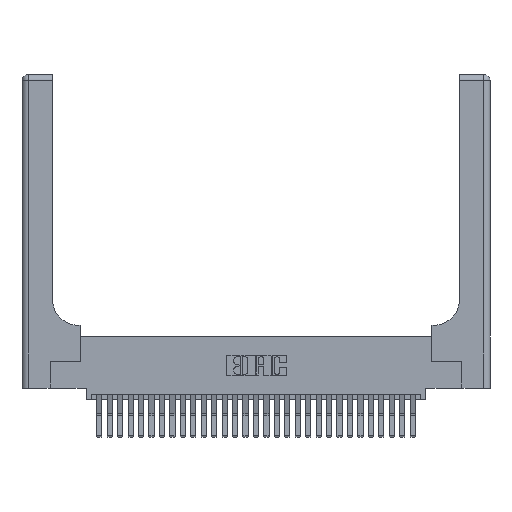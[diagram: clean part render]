
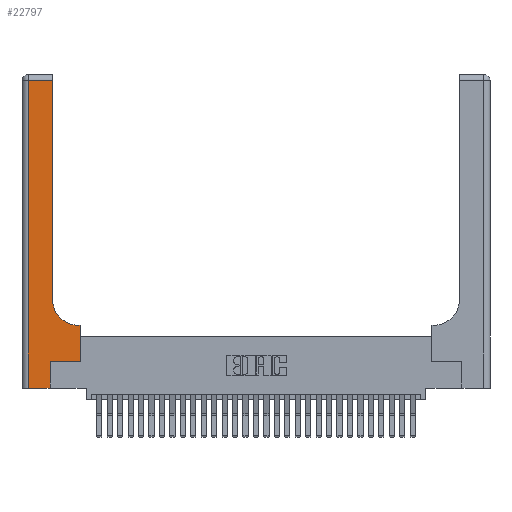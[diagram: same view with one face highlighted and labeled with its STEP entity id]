
A CAD part, top view. The second image highlights one B-rep face of the part: STEP entity #22797.
In plain terms, the highlighted planar face has unit normal (0, 0, 1).
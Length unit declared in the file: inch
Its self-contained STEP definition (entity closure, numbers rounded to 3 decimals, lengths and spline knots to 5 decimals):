
#344 = CARTESIAN_POINT ( 'NONE',  ( 0., 0., 0.37 ) ) ;
#548 = ORIENTED_EDGE ( 'NONE', *, *, #19670, .T. ) ;
#812 = VERTEX_POINT ( 'NONE', #15817 ) ;
#934 = EDGE_LOOP ( 'NONE', ( #19928, #30042, #25250, #17862, #3498, #10034, #18759, #548, #8731 ) ) ;
#982 = CARTESIAN_POINT ( 'NONE',  ( 0.06, 0., 0.37 ) ) ;
#1389 = PLANE ( 'NONE',  #23540 ) ;
#3209 = DIRECTION ( 'NONE',  ( -1., 0., 0. ) ) ;
#3498 = ORIENTED_EDGE ( 'NONE', *, *, #13362, .T. ) ;
#3582 = CARTESIAN_POINT ( 'NONE',  ( 0.06, 3., 0.37 ) ) ;
#3627 = VECTOR ( 'NONE', #20457, 39.37008 ) ;
#3640 = CARTESIAN_POINT ( 'NONE',  ( 0.269, 0.25, 0.37 ) ) ;
#3785 = EDGE_CURVE ( 'NONE', #4631, #9115, #19792, .T. ) ;
#3819 = DIRECTION ( 'NONE',  ( 0., 0., -1. ) ) ;
#4311 = LINE ( 'NONE', #3582, #24206 ) ;
#4631 = VERTEX_POINT ( 'NONE', #22765 ) ;
#6249 = CARTESIAN_POINT ( 'NONE',  ( 0.2915, 3., 0.37 ) ) ;
#6456 = VECTOR ( 'NONE', #13479, 39.37008 ) ;
#7193 = LINE ( 'NONE', #6249, #6456 ) ;
#7531 = DIRECTION ( 'NONE',  ( 1., 0., 0. ) ) ;
#7750 = CARTESIAN_POINT ( 'NONE',  ( 0.5585, 0.25, 0.37 ) ) ;
#7768 = LINE ( 'NONE', #13856, #19794 ) ;
#8546 = CARTESIAN_POINT ( 'NONE',  ( 0., 3., 0.37 ) ) ;
#8731 = ORIENTED_EDGE ( 'NONE', *, *, #23838, .T. ) ;
#8951 = EDGE_CURVE ( 'NONE', #19721, #30997, #13576, .T. ) ;
#9115 = VERTEX_POINT ( 'NONE', #20237 ) ;
#9307 = CARTESIAN_POINT ( 'NONE',  ( 0.5585, 0.25, 0.37 ) ) ;
#9394 = LINE ( 'NONE', #7750, #15759 ) ;
#9603 = DIRECTION ( 'NONE',  ( -1., 0., 0. ) ) ;
#10026 = LINE ( 'NONE', #3640, #3627 ) ;
#10034 = ORIENTED_EDGE ( 'NONE', *, *, #30050, .T. ) ;
#12058 = VECTOR ( 'NONE', #7531, 39.37008 ) ;
#12226 = VERTEX_POINT ( 'NONE', #26525 ) ;
#12600 = DIRECTION ( 'NONE',  ( 0., 0., -1. ) ) ;
#13362 = EDGE_CURVE ( 'NONE', #30997, #812, #7768, .T. ) ;
#13479 = DIRECTION ( 'NONE',  ( 0., 1., 0. ) ) ;
#13576 = LINE ( 'NONE', #344, #12058 ) ;
#13856 = CARTESIAN_POINT ( 'NONE',  ( 0.269, 0., 0.37 ) ) ;
#14422 = LINE ( 'NONE', #17595, #20812 ) ;
#14510 = CARTESIAN_POINT ( 'NONE',  ( 0.269, 0., 0.37 ) ) ;
#14690 = EDGE_CURVE ( 'NONE', #9115, #19721, #4311, .T. ) ;
#15759 = VECTOR ( 'NONE', #26989, 39.37008 ) ;
#15817 = CARTESIAN_POINT ( 'NONE',  ( 0.269, 0.25, 0.37 ) ) ;
#16929 = AXIS2_PLACEMENT_3D ( 'NONE', #26990, #12600, #29430 ) ;
#17595 = CARTESIAN_POINT ( 'NONE',  ( 0.2915, 0.6, 0.37 ) ) ;
#17862 = ORIENTED_EDGE ( 'NONE', *, *, #8951, .T. ) ;
#18698 = DIRECTION ( 'NONE',  ( 0., 1., 0. ) ) ;
#18759 = ORIENTED_EDGE ( 'NONE', *, *, #21905, .T. ) ;
#19037 = VECTOR ( 'NONE', #9603, 39.37008 ) ;
#19262 = CARTESIAN_POINT ( 'NONE',  ( 0., 2.94, 0.37 ) ) ;
#19670 = EDGE_CURVE ( 'NONE', #26735, #23711, #14422, .T. ) ;
#19721 = VERTEX_POINT ( 'NONE', #982 ) ;
#19758 = CARTESIAN_POINT ( 'NONE',  ( 0.5585, 0.6, 0.37 ) ) ;
#19792 = LINE ( 'NONE', #19262, #19037 ) ;
#19794 = VECTOR ( 'NONE', #18698, 39.37008 ) ;
#19928 = ORIENTED_EDGE ( 'NONE', *, *, #21048, .T. ) ;
#20237 = CARTESIAN_POINT ( 'NONE',  ( 0.06, 2.94, 0.37 ) ) ;
#20457 = DIRECTION ( 'NONE',  ( 1., 0., 0. ) ) ;
#20622 = DIRECTION ( 'NONE',  ( -1., 0., 0. ) ) ;
#20812 = VECTOR ( 'NONE', #3209, 39.37008 ) ;
#21048 = EDGE_CURVE ( 'NONE', #12226, #4631, #7193, .T. ) ;
#21905 = EDGE_CURVE ( 'NONE', #30317, #26735, #9394, .T. ) ;
#22283 = CIRCLE ( 'NONE', #16929, 0.25 ) ;
#22516 = FACE_OUTER_BOUND ( 'NONE', #934, .T. ) ;
#22765 = CARTESIAN_POINT ( 'NONE',  ( 0.2915, 2.94, 0.37 ) ) ;
#22795 = DIRECTION ( 'NONE',  ( 0., -1., 0. ) ) ;
#22797 = ADVANCED_FACE ( 'NONE', ( #22516 ), #1389, .F. ) ;
#23540 = AXIS2_PLACEMENT_3D ( 'NONE', #8546, #3819, #20622 ) ;
#23711 = VERTEX_POINT ( 'NONE', #26465 ) ;
#23838 = EDGE_CURVE ( 'NONE', #23711, #12226, #22283, .T. ) ;
#24206 = VECTOR ( 'NONE', #22795, 39.37008 ) ;
#25250 = ORIENTED_EDGE ( 'NONE', *, *, #14690, .T. ) ;
#26465 = CARTESIAN_POINT ( 'NONE',  ( 0.5415, 0.6, 0.37 ) ) ;
#26525 = CARTESIAN_POINT ( 'NONE',  ( 0.2915, 0.85, 0.37 ) ) ;
#26735 = VERTEX_POINT ( 'NONE', #19758 ) ;
#26989 = DIRECTION ( 'NONE',  ( 0., 1., 0. ) ) ;
#26990 = CARTESIAN_POINT ( 'NONE',  ( 0.5415, 0.85, 0.37 ) ) ;
#29430 = DIRECTION ( 'NONE',  ( 1., 0., 0. ) ) ;
#30042 = ORIENTED_EDGE ( 'NONE', *, *, #3785, .T. ) ;
#30050 = EDGE_CURVE ( 'NONE', #812, #30317, #10026, .T. ) ;
#30317 = VERTEX_POINT ( 'NONE', #9307 ) ;
#30997 = VERTEX_POINT ( 'NONE', #14510 ) ;
